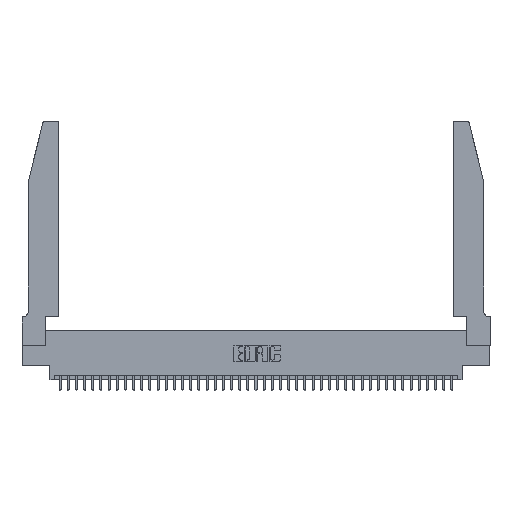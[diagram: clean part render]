
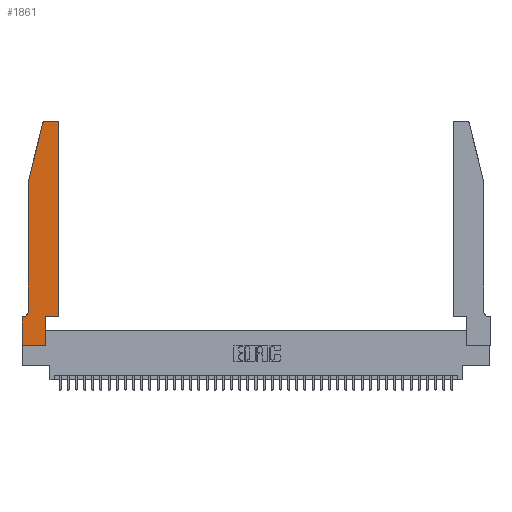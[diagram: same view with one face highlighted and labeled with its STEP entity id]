
A CAD part, top view. The second image highlights one B-rep face of the part: STEP entity #1861.
In plain terms, the highlighted planar face has unit normal (0, 0, 1).
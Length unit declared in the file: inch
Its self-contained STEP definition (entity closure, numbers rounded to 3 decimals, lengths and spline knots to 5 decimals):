
#142 = CARTESIAN_POINT ( 'NONE',  ( 0., 0., 0.37 ) ) ;
#192 = EDGE_LOOP ( 'NONE', ( #18605, #28538, #9829, #9778, #25983, #4519, #3918, #15520, #4546, #9098, #10344, #34451 ) ) ;
#406 = LINE ( 'NONE', #6655, #13787 ) ;
#667 = CIRCLE ( 'NONE', #7617, 0.03 ) ;
#1180 = DIRECTION ( 'NONE',  ( 0., 0., 1. ) ) ;
#1405 = EDGE_CURVE ( 'NONE', #40249, #11949, #23277, .T. ) ;
#1787 = VECTOR ( 'NONE', #18959, 39.37008 ) ;
#1861 = ADVANCED_FACE ( 'NONE', ( #41618 ), #12674, .T. ) ;
#1870 = DIRECTION ( 'NONE',  ( 0., -1., 0. ) ) ;
#2329 = VERTEX_POINT ( 'NONE', #29613 ) ;
#2749 = VECTOR ( 'NONE', #23539, 39.37008 ) ;
#3444 = DIRECTION ( 'NONE',  ( 0., -1., 0. ) ) ;
#3472 = VECTOR ( 'NONE', #34968, 39.37008 ) ;
#3918 = ORIENTED_EDGE ( 'NONE', *, *, #10945, .T. ) ;
#4199 = CARTESIAN_POINT ( 'NONE',  ( 0.0755, 2., 0.37 ) ) ;
#4519 = ORIENTED_EDGE ( 'NONE', *, *, #35730, .T. ) ;
#4546 = ORIENTED_EDGE ( 'NONE', *, *, #30200, .T. ) ;
#4722 = CARTESIAN_POINT ( 'NONE',  ( 0.25487, 2.72718, 0.37 ) ) ;
#6515 = DIRECTION ( 'NONE',  ( -1., 0., 0. ) ) ;
#6655 = CARTESIAN_POINT ( 'NONE',  ( 0.0755, 0.35, 0.37 ) ) ;
#7284 = CARTESIAN_POINT ( 'NONE',  ( 0.2865, 0.35, 0.37 ) ) ;
#7617 = AXIS2_PLACEMENT_3D ( 'NONE', #20856, #1180, #17076 ) ;
#7743 = CARTESIAN_POINT ( 'NONE',  ( 0., 0.35, 0.37 ) ) ;
#8433 = LINE ( 'NONE', #9394, #42254 ) ;
#8838 = CARTESIAN_POINT ( 'NONE',  ( 0.284, 2.72, 0.37 ) ) ;
#9098 = ORIENTED_EDGE ( 'NONE', *, *, #38278, .T. ) ;
#9394 = CARTESIAN_POINT ( 'NONE',  ( 0.2605, 2.75, 0.37 ) ) ;
#9778 = ORIENTED_EDGE ( 'NONE', *, *, #21938, .T. ) ;
#9829 = ORIENTED_EDGE ( 'NONE', *, *, #30704, .T. ) ;
#10344 = ORIENTED_EDGE ( 'NONE', *, *, #17797, .T. ) ;
#10656 = EDGE_CURVE ( 'NONE', #34169, #29639, #8433, .T. ) ;
#10945 = EDGE_CURVE ( 'NONE', #14504, #40249, #37109, .T. ) ;
#10977 = LINE ( 'NONE', #19287, #15561 ) ;
#11949 = VERTEX_POINT ( 'NONE', #35385 ) ;
#12674 = PLANE ( 'NONE',  #32982 ) ;
#12736 = CARTESIAN_POINT ( 'NONE',  ( 0., 0., 0.37 ) ) ;
#13787 = VECTOR ( 'NONE', #6515, 39.37008 ) ;
#14504 = VERTEX_POINT ( 'NONE', #7743 ) ;
#14643 = CIRCLE ( 'NONE', #38626, 0.03 ) ;
#14728 = DIRECTION ( 'NONE',  ( -1., 0., 0. ) ) ;
#15520 = ORIENTED_EDGE ( 'NONE', *, *, #1405, .T. ) ;
#15561 = VECTOR ( 'NONE', #28607, 39.37008 ) ;
#15863 = VERTEX_POINT ( 'NONE', #4722 ) ;
#15938 = CARTESIAN_POINT ( 'NONE',  ( 0.284, 2.75, 0.37 ) ) ;
#16441 = EDGE_CURVE ( 'NONE', #29639, #15863, #14643, .T. ) ;
#16617 = EDGE_CURVE ( 'NONE', #27990, #2329, #32627, .T. ) ;
#17076 = DIRECTION ( 'NONE',  ( 1., 0., 0. ) ) ;
#17434 = AXIS2_PLACEMENT_3D ( 'NONE', #21511, #21081, #14728 ) ;
#17530 = EDGE_CURVE ( 'NONE', #18124, #34169, #667, .T. ) ;
#17797 = EDGE_CURVE ( 'NONE', #37964, #18124, #10977, .T. ) ;
#18124 = VERTEX_POINT ( 'NONE', #25085 ) ;
#18188 = LINE ( 'NONE', #4199, #20719 ) ;
#18605 = ORIENTED_EDGE ( 'NONE', *, *, #10656, .T. ) ;
#18959 = DIRECTION ( 'NONE',  ( 1., 0., 0. ) ) ;
#19065 = CARTESIAN_POINT ( 'NONE',  ( 0.0755, 2., 0.37 ) ) ;
#19079 = CARTESIAN_POINT ( 'NONE',  ( 0.4205, 2.75, 0.37 ) ) ;
#19281 = LINE ( 'NONE', #22123, #1787 ) ;
#19287 = CARTESIAN_POINT ( 'NONE',  ( 0.4505, 0.35, 0.37 ) ) ;
#20719 = VECTOR ( 'NONE', #1870, 39.37008 ) ;
#20856 = CARTESIAN_POINT ( 'NONE',  ( 0.4205, 2.72, 0.37 ) ) ;
#21081 = DIRECTION ( 'NONE',  ( 0., 0., -1. ) ) ;
#21511 = CARTESIAN_POINT ( 'NONE',  ( 0.0055, 0.42, 0.37 ) ) ;
#21938 = EDGE_CURVE ( 'NONE', #31438, #27990, #18188, .T. ) ;
#22123 = CARTESIAN_POINT ( 'NONE',  ( 0.4505, 0.35, 0.37 ) ) ;
#22261 = DIRECTION ( 'NONE',  ( 0., 1., 0. ) ) ;
#23277 = LINE ( 'NONE', #142, #2749 ) ;
#23539 = DIRECTION ( 'NONE',  ( 1., 0., 0. ) ) ;
#23999 = DIRECTION ( 'NONE',  ( 1., 0., 0. ) ) ;
#24077 = CARTESIAN_POINT ( 'NONE',  ( 0.0755, 0.42, 0.37 ) ) ;
#25085 = CARTESIAN_POINT ( 'NONE',  ( 0.4505, 2.72, 0.37 ) ) ;
#25983 = ORIENTED_EDGE ( 'NONE', *, *, #16617, .T. ) ;
#26365 = VECTOR ( 'NONE', #3444, 39.37008 ) ;
#27990 = VERTEX_POINT ( 'NONE', #24077 ) ;
#28186 = CARTESIAN_POINT ( 'NONE',  ( 0.0755, 2., 0.37 ) ) ;
#28480 = CARTESIAN_POINT ( 'NONE',  ( 0., 0.35, 0.37 ) ) ;
#28538 = ORIENTED_EDGE ( 'NONE', *, *, #16441, .T. ) ;
#28607 = DIRECTION ( 'NONE',  ( 0., 1., 0. ) ) ;
#28632 = DIRECTION ( 'NONE',  ( 0., 0., 1. ) ) ;
#28909 = DIRECTION ( 'NONE',  ( 1., 0., 0. ) ) ;
#29613 = CARTESIAN_POINT ( 'NONE',  ( 0.0055, 0.35, 0.37 ) ) ;
#29639 = VERTEX_POINT ( 'NONE', #15938 ) ;
#30200 = EDGE_CURVE ( 'NONE', #11949, #34376, #40386, .T. ) ;
#30704 = EDGE_CURVE ( 'NONE', #15863, #31438, #34718, .T. ) ;
#31438 = VERTEX_POINT ( 'NONE', #28186 ) ;
#32627 = CIRCLE ( 'NONE', #17434, 0.07 ) ;
#32968 = CARTESIAN_POINT ( 'NONE',  ( 0., 0., 0.37 ) ) ;
#32982 = AXIS2_PLACEMENT_3D ( 'NONE', #28480, #28632, #28909 ) ;
#34169 = VERTEX_POINT ( 'NONE', #19079 ) ;
#34376 = VERTEX_POINT ( 'NONE', #7284 ) ;
#34451 = ORIENTED_EDGE ( 'NONE', *, *, #17530, .T. ) ;
#34558 = CARTESIAN_POINT ( 'NONE',  ( 0.4505, 0.35, 0.37 ) ) ;
#34718 = LINE ( 'NONE', #19065, #3472 ) ;
#34968 = DIRECTION ( 'NONE',  ( -0.239, -0.971, 0. ) ) ;
#35299 = VECTOR ( 'NONE', #22261, 39.37008 ) ;
#35385 = CARTESIAN_POINT ( 'NONE',  ( 0.2865, 0., 0.37 ) ) ;
#35730 = EDGE_CURVE ( 'NONE', #2329, #14504, #406, .T. ) ;
#37109 = LINE ( 'NONE', #12736, #26365 ) ;
#37964 = VERTEX_POINT ( 'NONE', #34558 ) ;
#38278 = EDGE_CURVE ( 'NONE', #34376, #37964, #19281, .T. ) ;
#38475 = DIRECTION ( 'NONE',  ( -1., 0., 0. ) ) ;
#38626 = AXIS2_PLACEMENT_3D ( 'NONE', #8838, #39177, #23999 ) ;
#39177 = DIRECTION ( 'NONE',  ( 0., 0., 1. ) ) ;
#40249 = VERTEX_POINT ( 'NONE', #32968 ) ;
#40386 = LINE ( 'NONE', #41832, #35299 ) ;
#41618 = FACE_OUTER_BOUND ( 'NONE', #192, .T. ) ;
#41832 = CARTESIAN_POINT ( 'NONE',  ( 0.2865, 0.35, 0.37 ) ) ;
#42254 = VECTOR ( 'NONE', #38475, 39.37008 ) ;
